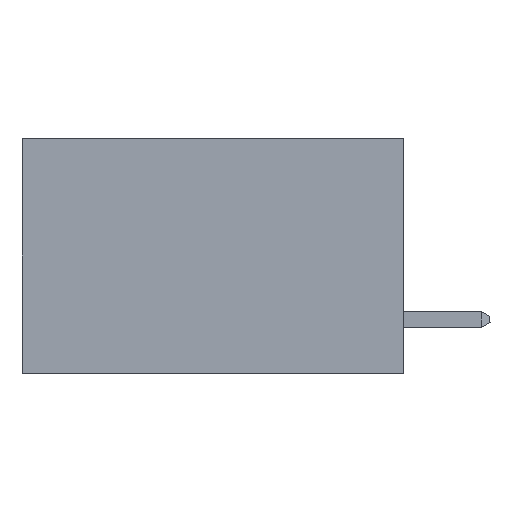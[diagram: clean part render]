
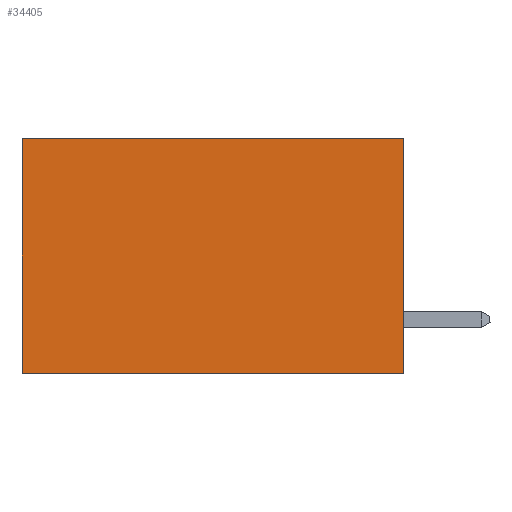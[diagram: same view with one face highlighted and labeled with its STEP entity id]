
A CAD part, left-side view. The second image highlights one B-rep face of the part: STEP entity #34405.
In plain terms, the highlighted planar face has unit normal (-1, 0, 0).
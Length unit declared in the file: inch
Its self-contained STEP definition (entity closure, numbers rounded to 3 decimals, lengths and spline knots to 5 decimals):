
#1100 = CARTESIAN_POINT ( 'NONE',  ( 0.2875, 0.6, 0. ) ) ;
#3169 = LINE ( 'NONE', #19676, #40091 ) ;
#3802 = CARTESIAN_POINT ( 'NONE',  ( 0.2875, 0.6, 0. ) ) ;
#4600 = EDGE_CURVE ( 'NONE', #34128, #16556, #3169, .T. ) ;
#5261 = CARTESIAN_POINT ( 'NONE',  ( 0.2875, 0.6, -0.37 ) ) ;
#7465 = DIRECTION ( 'NONE',  ( 0., 1., 0. ) ) ;
#8732 = LINE ( 'NONE', #21971, #13890 ) ;
#10602 = FACE_OUTER_BOUND ( 'NONE', #26085, .T. ) ;
#11350 = ORIENTED_EDGE ( 'NONE', *, *, #18675, .T. ) ;
#11367 = DIRECTION ( 'NONE',  ( 0., 0., -1. ) ) ;
#12020 = PLANE ( 'NONE',  #17211 ) ;
#12122 = VERTEX_POINT ( 'NONE', #25876 ) ;
#13890 = VECTOR ( 'NONE', #41672, 39.37008 ) ;
#16556 = VERTEX_POINT ( 'NONE', #5261 ) ;
#17211 = AXIS2_PLACEMENT_3D ( 'NONE', #38055, #22025, #28319 ) ;
#18675 = EDGE_CURVE ( 'NONE', #35305, #16556, #38676, .T. ) ;
#19171 = ORIENTED_EDGE ( 'NONE', *, *, #23944, .T. ) ;
#19676 = CARTESIAN_POINT ( 'NONE',  ( 0.2875, 0., -0.37 ) ) ;
#20947 = VECTOR ( 'NONE', #36171, 39.37008 ) ;
#21971 = CARTESIAN_POINT ( 'NONE',  ( 0.2875, 0., 0. ) ) ;
#22025 = DIRECTION ( 'NONE',  ( 1., 0., 0. ) ) ;
#23205 = CARTESIAN_POINT ( 'NONE',  ( 0.2875, 0., -0.37 ) ) ;
#23797 = ORIENTED_EDGE ( 'NONE', *, *, #32308, .F. ) ;
#23944 = EDGE_CURVE ( 'NONE', #12122, #35305, #26043, .T. ) ;
#25876 = CARTESIAN_POINT ( 'NONE',  ( 0.2875, 0., 0. ) ) ;
#26043 = LINE ( 'NONE', #39466, #20947 ) ;
#26085 = EDGE_LOOP ( 'NONE', ( #11350, #38033, #23797, #19171 ) ) ;
#28319 = DIRECTION ( 'NONE',  ( 0., 0., -1. ) ) ;
#32308 = EDGE_CURVE ( 'NONE', #12122, #34128, #8732, .T. ) ;
#33020 = VECTOR ( 'NONE', #11367, 39.37008 ) ;
#34128 = VERTEX_POINT ( 'NONE', #23205 ) ;
#34405 = ADVANCED_FACE ( 'NONE', ( #10602 ), #12020, .F. ) ;
#35305 = VERTEX_POINT ( 'NONE', #3802 ) ;
#36171 = DIRECTION ( 'NONE',  ( 0., 1., 0. ) ) ;
#38033 = ORIENTED_EDGE ( 'NONE', *, *, #4600, .F. ) ;
#38055 = CARTESIAN_POINT ( 'NONE',  ( 0.2875, 0., 0. ) ) ;
#38676 = LINE ( 'NONE', #1100, #33020 ) ;
#39466 = CARTESIAN_POINT ( 'NONE',  ( 0.2875, 0., 0. ) ) ;
#40091 = VECTOR ( 'NONE', #7465, 39.37008 ) ;
#41672 = DIRECTION ( 'NONE',  ( 0., 0., -1. ) ) ;
